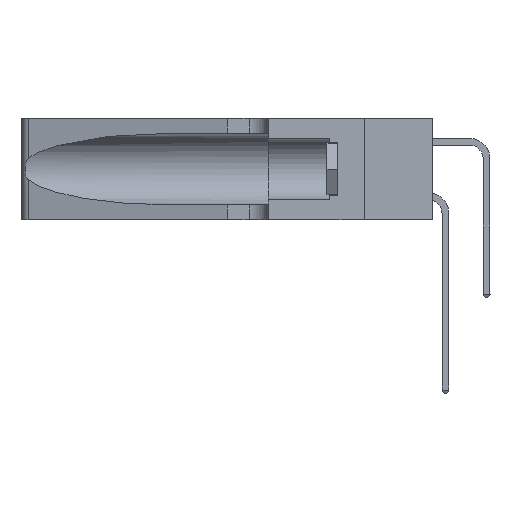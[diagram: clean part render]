
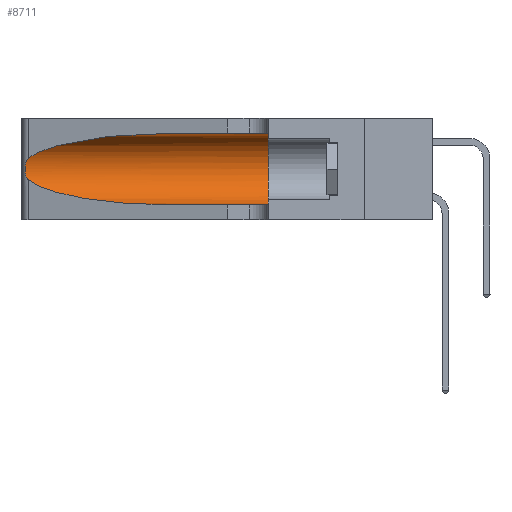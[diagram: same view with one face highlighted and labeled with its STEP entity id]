
A CAD part, left-side view. The second image highlights one B-rep face of the part: STEP entity #8711.
In plain terms, the highlighted cylindrical face has radius 3.308 mm (diameter 6.617 mm), a partial arc.
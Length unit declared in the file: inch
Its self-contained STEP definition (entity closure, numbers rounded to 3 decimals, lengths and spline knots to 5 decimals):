
#220 = VECTOR ( 'NONE', #4617, 39.37008 ) ;
#790 = ORIENTED_EDGE ( 'NONE', *, *, #23026, .T. ) ;
#1758 = VERTEX_POINT ( 'NONE', #15004 ) ;
#1891 = CARTESIAN_POINT ( 'NONE',  ( 0.26017, 1.23833, 0.17102 ) ) ;
#2371 = VERTEX_POINT ( 'NONE', #2710 ) ;
#2382 = CYLINDRICAL_SURFACE ( 'NONE', #15357, 0.13025 ) ;
#2710 = CARTESIAN_POINT ( 'NONE',  ( 0.25487, 1.22718, 0.22369 ) ) ;
#3320 = CARTESIAN_POINT ( 'NONE',  ( 0.1305, 0.72297, 0.31525 ) ) ;
#3903 = DIRECTION ( 'NONE',  ( 0., 1., 0. ) ) ;
#3913 = VERTEX_POINT ( 'NONE', #22315 ) ;
#4015 = EDGE_CURVE ( 'NONE', #24533, #29810, #22595, .T. ) ;
#4270 = ORIENTED_EDGE ( 'NONE', *, *, #27942, .T. ) ;
#4341 = CARTESIAN_POINT ( 'NONE',  ( 0.25789, 1.23486, 0.15765 ) ) ;
#4617 = DIRECTION ( 'NONE',  ( 0., -1., 0. ) ) ;
#5127 = CARTESIAN_POINT ( 'NONE',  ( 0.18966, 0.96281, 0.05475 ) ) ;
#5719 = CARTESIAN_POINT ( 'NONE',  ( 0.18966, 0.96281, 0.31525 ) ) ;
#6749 = CARTESIAN_POINT ( 'NONE',  ( 0.25555, 1.22993, 0.14849 ) ) ;
#8711 = ADVANCED_FACE ( 'NONE', ( #15043 ), #2382, .F. ) ;
#8867 = B_SPLINE_CURVE_WITH_KNOTS ( 'NONE', 3,
 ( #29761, #27387, #25295, #11400, #27581, #13785, #29851, #16143, #1891, #18486, #4341, #20835, #6749, #23104 ),
 .UNSPECIFIED., .F., .F.,
 ( 4, 2, 2, 2, 2, 2, 4 ),
 ( 0., 0.00027, 0.00053, 0.00107, 0.0016, 0.00187, 0.00214 ),
 .UNSPECIFIED. ) ;
#10584 = DIRECTION ( 'NONE',  ( 0., 0., -1. ) ) ;
#10860 = ORIENTED_EDGE ( 'NONE', *, *, #19018, .T. ) ;
#11400 = CARTESIAN_POINT ( 'NONE',  ( 0.25787, 1.23484, 0.2124 ) ) ;
#12877 = CARTESIAN_POINT ( 'NONE',  ( 0.25487, 1.22718, 0.22369 ) ) ;
#12941 = LINE ( 'NONE', #23373, #220 ) ;
#13785 = CARTESIAN_POINT ( 'NONE',  ( 0.26018, 1.23835, 0.19895 ) ) ;
#14177 = EDGE_LOOP ( 'NONE', ( #4270, #10860, #790, #16297, #26963, #20617 ) ) ;
#15004 = CARTESIAN_POINT ( 'NONE',  ( 0.1305, 0.72297, 0.31525 ) ) ;
#15043 = FACE_OUTER_BOUND ( 'NONE', #14177, .T. ) ;
#15327 = DIRECTION ( 'NONE',  ( 0., -1., 0. ) ) ;
#15357 = AXIS2_PLACEMENT_3D ( 'NONE', #29065, #15327, #10584 ) ;
#16143 = CARTESIAN_POINT ( 'NONE',  ( 0.26075, 1.23896, 0.178 ) ) ;
#16297 = ORIENTED_EDGE ( 'NONE', *, *, #27146, .T. ) ;
#16926 = CARTESIAN_POINT ( 'NONE',  ( 0.25487, 1.22718, 0.14631 ) ) ;
#18049 = CARTESIAN_POINT ( 'NONE',  ( 0.1305, 0.35, 0.185 ) ) ;
#18486 = CARTESIAN_POINT ( 'NONE',  ( 0.25856, 1.23593, 0.16098 ) ) ;
#19018 = EDGE_CURVE ( 'NONE', #2371, #27836, #8867, .T. ) ;
#19263 = CARTESIAN_POINT ( 'NONE',  ( 0.2373, 1.15595, 0.08982 ) ) ;
#20396 = DIRECTION ( 'NONE',  ( 0., 0., 1. ) ) ;
#20617 = ORIENTED_EDGE ( 'NONE', *, *, #29910, .F. ) ;
#20721 =( BOUNDED_CURVE ( )  B_SPLINE_CURVE ( 3, ( #3320, #5719, #26723, #12877 ),
 .UNSPECIFIED., .F., .F. ) 
 B_SPLINE_CURVE_WITH_KNOTS ( ( 4, 4 ),
 ( 1.5708, 2.84003 ),
 .UNSPECIFIED. ) 
 CURVE ( )  GEOMETRIC_REPRESENTATION_ITEM ( )  RATIONAL_B_SPLINE_CURVE ( ( 1., 0.87, 0.87, 1. ) ) 
 REPRESENTATION_ITEM ( '' )  );
#20835 = CARTESIAN_POINT ( 'NONE',  ( 0.25639, 1.23186, 0.15144 ) ) ;
#21607 = CARTESIAN_POINT ( 'NONE',  ( 0.1305, 0.72297, 0.05475 ) ) ;
#21620 = VECTOR ( 'NONE', #23458, 39.37008 ) ;
#22315 = CARTESIAN_POINT ( 'NONE',  ( 0.1305, 0.72297, 0.05475 ) ) ;
#22328 = LINE ( 'NONE', #25760, #21620 ) ;
#22595 = CIRCLE ( 'NONE', #24927, 0.13025 ) ;
#22906 =( BOUNDED_CURVE ( )  B_SPLINE_CURVE ( 3, ( #16926, #19263, #5127, #21607 ),
 .UNSPECIFIED., .F., .T. ) 
 B_SPLINE_CURVE_WITH_KNOTS ( ( 4, 4 ),
 ( 3.44316, 4.71239 ),
 .UNSPECIFIED. ) 
 CURVE ( )  GEOMETRIC_REPRESENTATION_ITEM ( )  RATIONAL_B_SPLINE_CURVE ( ( 1., 0.87, 0.87, 1. ) ) 
 REPRESENTATION_ITEM ( '' )  );
#23026 = EDGE_CURVE ( 'NONE', #27836, #3913, #22906, .T. ) ;
#23104 = CARTESIAN_POINT ( 'NONE',  ( 0.25487, 1.22718, 0.14631 ) ) ;
#23373 = CARTESIAN_POINT ( 'NONE',  ( 0.1305, 1.61858, 0.31525 ) ) ;
#23458 = DIRECTION ( 'NONE',  ( 0., -1., 0. ) ) ;
#24533 = VERTEX_POINT ( 'NONE', #27153 ) ;
#24927 = AXIS2_PLACEMENT_3D ( 'NONE', #18049, #3903, #20396 ) ;
#25295 = CARTESIAN_POINT ( 'NONE',  ( 0.25639, 1.23184, 0.21858 ) ) ;
#25760 = CARTESIAN_POINT ( 'NONE',  ( 0.1305, 1.61858, 0.05475 ) ) ;
#26723 = CARTESIAN_POINT ( 'NONE',  ( 0.2373, 1.15595, 0.28018 ) ) ;
#26963 = ORIENTED_EDGE ( 'NONE', *, *, #4015, .F. ) ;
#27146 = EDGE_CURVE ( 'NONE', #3913, #29810, #22328, .T. ) ;
#27153 = CARTESIAN_POINT ( 'NONE',  ( 0.1305, 0.35, 0.31525 ) ) ;
#27387 = CARTESIAN_POINT ( 'NONE',  ( 0.25555, 1.22994, 0.2215 ) ) ;
#27581 = CARTESIAN_POINT ( 'NONE',  ( 0.25854, 1.2359, 0.20912 ) ) ;
#27836 = VERTEX_POINT ( 'NONE', #28615 ) ;
#27942 = EDGE_CURVE ( 'NONE', #1758, #2371, #20721, .T. ) ;
#28615 = CARTESIAN_POINT ( 'NONE',  ( 0.25487, 1.22718, 0.14631 ) ) ;
#29065 = CARTESIAN_POINT ( 'NONE',  ( 0.1305, 1.61858, 0.185 ) ) ;
#29735 = CARTESIAN_POINT ( 'NONE',  ( 0.1305, 0.35, 0.05475 ) ) ;
#29761 = CARTESIAN_POINT ( 'NONE',  ( 0.25487, 1.22718, 0.22369 ) ) ;
#29810 = VERTEX_POINT ( 'NONE', #29735 ) ;
#29851 = CARTESIAN_POINT ( 'NONE',  ( 0.26075, 1.23896, 0.19203 ) ) ;
#29910 = EDGE_CURVE ( 'NONE', #1758, #24533, #12941, .T. ) ;
